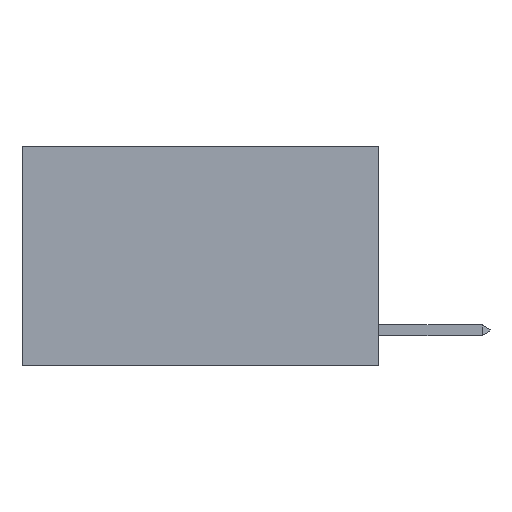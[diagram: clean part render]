
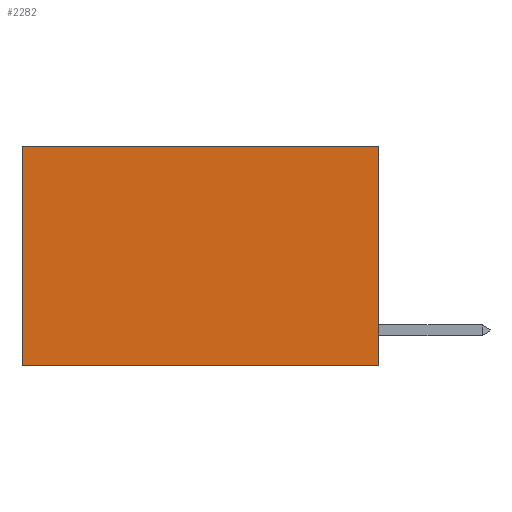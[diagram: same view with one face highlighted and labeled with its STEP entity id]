
A CAD part, left-side view. The second image highlights one B-rep face of the part: STEP entity #2282.
In plain terms, the highlighted planar face has unit normal (-1, 0, 0).
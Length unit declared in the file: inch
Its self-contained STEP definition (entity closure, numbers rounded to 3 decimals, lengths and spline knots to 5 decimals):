
#1433 = DIRECTION ( 'NONE',  ( 0., 1., 0. ) ) ;
#1550 = CARTESIAN_POINT ( 'NONE',  ( 0.2625, 0., 0. ) ) ;
#2282 = ADVANCED_FACE ( 'NONE', ( #12535 ), #3330, .F. ) ;
#2928 = ORIENTED_EDGE ( 'NONE', *, *, #10670, .T. ) ;
#3330 = PLANE ( 'NONE',  #4495 ) ;
#4495 = AXIS2_PLACEMENT_3D ( 'NONE', #1550, #8801, #8530 ) ;
#4820 = EDGE_CURVE ( 'NONE', #15175, #12846, #5896, .T. ) ;
#5813 = VERTEX_POINT ( 'NONE', #12413 ) ;
#5896 = LINE ( 'NONE', #10827, #16486 ) ;
#6075 = EDGE_LOOP ( 'NONE', ( #7043, #9863, #7312, #2928 ) ) ;
#6510 = VECTOR ( 'NONE', #9010, 39.37008 ) ;
#6938 = LINE ( 'NONE', #7642, #6510 ) ;
#7043 = ORIENTED_EDGE ( 'NONE', *, *, #11042, .T. ) ;
#7253 = CARTESIAN_POINT ( 'NONE',  ( 0.2625, 0., 0. ) ) ;
#7312 = ORIENTED_EDGE ( 'NONE', *, *, #4820, .F. ) ;
#7642 = CARTESIAN_POINT ( 'NONE',  ( 0.2625, 0.6, 0. ) ) ;
#7654 = VECTOR ( 'NONE', #1433, 39.37008 ) ;
#7797 = CARTESIAN_POINT ( 'NONE',  ( 0.2625, 0.6, -0.37 ) ) ;
#8483 = CARTESIAN_POINT ( 'NONE',  ( 0.2625, 0., 0. ) ) ;
#8530 = DIRECTION ( 'NONE',  ( 0., 0., -1. ) ) ;
#8532 = EDGE_CURVE ( 'NONE', #12846, #9515, #13346, .T. ) ;
#8801 = DIRECTION ( 'NONE',  ( 1., 0., 0. ) ) ;
#9010 = DIRECTION ( 'NONE',  ( 0., 0., -1. ) ) ;
#9515 = VERTEX_POINT ( 'NONE', #7797 ) ;
#9863 = ORIENTED_EDGE ( 'NONE', *, *, #8532, .F. ) ;
#10670 = EDGE_CURVE ( 'NONE', #15175, #5813, #11655, .T. ) ;
#10827 = CARTESIAN_POINT ( 'NONE',  ( 0.2625, 0., 0. ) ) ;
#11042 = EDGE_CURVE ( 'NONE', #5813, #9515, #6938, .T. ) ;
#11655 = LINE ( 'NONE', #8483, #7654 ) ;
#12413 = CARTESIAN_POINT ( 'NONE',  ( 0.2625, 0.6, 0. ) ) ;
#12535 = FACE_OUTER_BOUND ( 'NONE', #6075, .T. ) ;
#12789 = CARTESIAN_POINT ( 'NONE',  ( 0.2625, 0., -0.37 ) ) ;
#12846 = VERTEX_POINT ( 'NONE', #13040 ) ;
#13040 = CARTESIAN_POINT ( 'NONE',  ( 0.2625, 0., -0.37 ) ) ;
#13346 = LINE ( 'NONE', #12789, #15582 ) ;
#13387 = DIRECTION ( 'NONE',  ( 0., 0., -1. ) ) ;
#15175 = VERTEX_POINT ( 'NONE', #7253 ) ;
#15391 = DIRECTION ( 'NONE',  ( 0., 1., 0. ) ) ;
#15582 = VECTOR ( 'NONE', #15391, 39.37008 ) ;
#16486 = VECTOR ( 'NONE', #13387, 39.37008 ) ;
